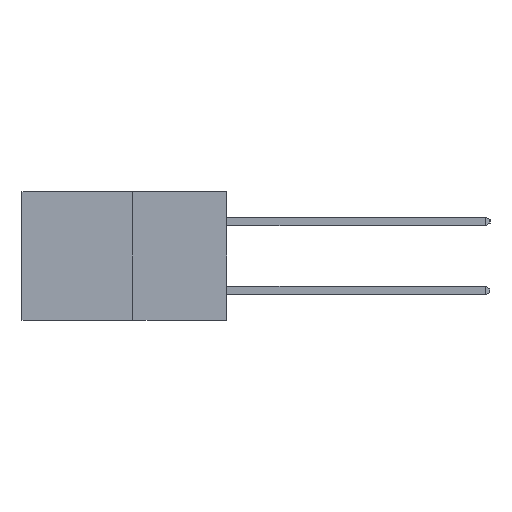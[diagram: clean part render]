
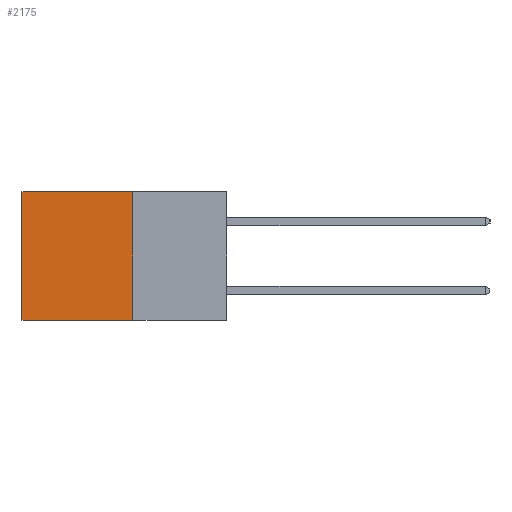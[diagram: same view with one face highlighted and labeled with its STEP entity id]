
A CAD part, left-side view. The second image highlights one B-rep face of the part: STEP entity #2175.
In plain terms, the highlighted planar face has unit normal (-1, 0, 0).
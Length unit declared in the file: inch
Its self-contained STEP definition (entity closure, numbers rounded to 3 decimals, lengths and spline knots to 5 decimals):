
#618 = CARTESIAN_POINT ( 'NONE',  ( 0.277, 0.27, 0. ) ) ;
#633 = VECTOR ( 'NONE', #3052, 39.37008 ) ;
#1648 = VECTOR ( 'NONE', #6811, 39.37008 ) ;
#2144 = EDGE_LOOP ( 'NONE', ( #4039, #4890, #5636, #2631 ) ) ;
#2175 = ADVANCED_FACE ( 'NONE', ( #2996 ), #3643, .F. ) ;
#2631 = ORIENTED_EDGE ( 'NONE', *, *, #4669, .T. ) ;
#2738 = CARTESIAN_POINT ( 'NONE',  ( 0.277, 0.59, 0. ) ) ;
#2996 = FACE_OUTER_BOUND ( 'NONE', #2144, .T. ) ;
#3052 = DIRECTION ( 'NONE',  ( 0., 1., 0. ) ) ;
#3215 = AXIS2_PLACEMENT_3D ( 'NONE', #8582, #5082, #3365 ) ;
#3365 = DIRECTION ( 'NONE',  ( 0., 0., -1. ) ) ;
#3547 = LINE ( 'NONE', #618, #9970 ) ;
#3643 = PLANE ( 'NONE',  #3215 ) ;
#3759 = CARTESIAN_POINT ( 'NONE',  ( 0.277, 0.59, -0.37 ) ) ;
#4039 = ORIENTED_EDGE ( 'NONE', *, *, #5041, .T. ) ;
#4142 = DIRECTION ( 'NONE',  ( 0., 0., -1. ) ) ;
#4448 = CARTESIAN_POINT ( 'NONE',  ( 0.277, 0.27, 0. ) ) ;
#4669 = EDGE_CURVE ( 'NONE', #8314, #9657, #3547, .T. ) ;
#4811 = CARTESIAN_POINT ( 'NONE',  ( 0.277, 0.27, -0.37 ) ) ;
#4890 = ORIENTED_EDGE ( 'NONE', *, *, #7776, .F. ) ;
#5041 = EDGE_CURVE ( 'NONE', #9657, #7057, #5936, .T. ) ;
#5082 = DIRECTION ( 'NONE',  ( 1., 0., 0. ) ) ;
#5527 = DIRECTION ( 'NONE',  ( 0., 1., 0. ) ) ;
#5636 = ORIENTED_EDGE ( 'NONE', *, *, #9463, .F. ) ;
#5936 = LINE ( 'NONE', #9291, #1648 ) ;
#6730 = VECTOR ( 'NONE', #4142, 39.37008 ) ;
#6811 = DIRECTION ( 'NONE',  ( 0., 0., -1. ) ) ;
#6893 = LINE ( 'NONE', #7063, #633 ) ;
#7057 = VERTEX_POINT ( 'NONE', #3759 ) ;
#7063 = CARTESIAN_POINT ( 'NONE',  ( 0.277, 0.27, -0.37 ) ) ;
#7776 = EDGE_CURVE ( 'NONE', #9350, #7057, #6893, .T. ) ;
#8314 = VERTEX_POINT ( 'NONE', #4448 ) ;
#8582 = CARTESIAN_POINT ( 'NONE',  ( 0.277, 0.27, -0.37 ) ) ;
#8916 = LINE ( 'NONE', #9758, #6730 ) ;
#9291 = CARTESIAN_POINT ( 'NONE',  ( 0.277, 0.59, -0.37 ) ) ;
#9350 = VERTEX_POINT ( 'NONE', #4811 ) ;
#9463 = EDGE_CURVE ( 'NONE', #8314, #9350, #8916, .T. ) ;
#9657 = VERTEX_POINT ( 'NONE', #2738 ) ;
#9758 = CARTESIAN_POINT ( 'NONE',  ( 0.277, 0.27, -0.37 ) ) ;
#9970 = VECTOR ( 'NONE', #5527, 39.37008 ) ;
